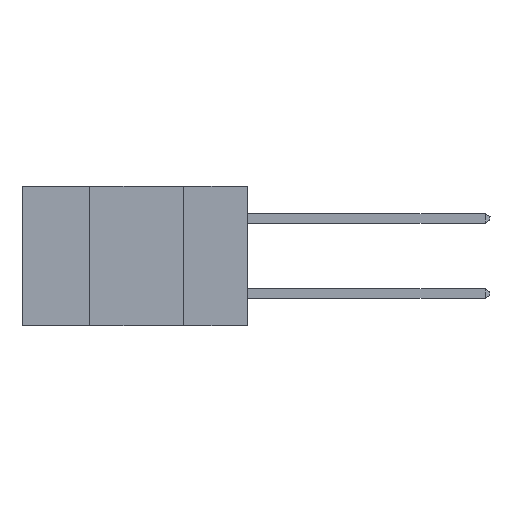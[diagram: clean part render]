
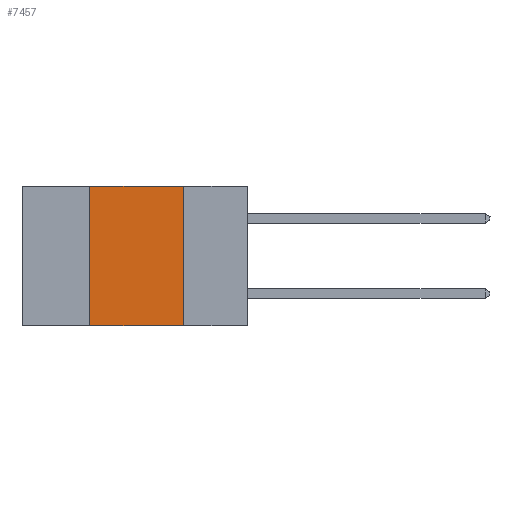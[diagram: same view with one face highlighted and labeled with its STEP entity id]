
A CAD part, left-side view. The second image highlights one B-rep face of the part: STEP entity #7457.
In plain terms, the highlighted planar face has unit normal (-1, 0, 0).
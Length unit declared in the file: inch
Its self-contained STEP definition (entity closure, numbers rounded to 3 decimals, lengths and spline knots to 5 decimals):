
#101 = AXIS2_PLACEMENT_3D ( 'NONE', #11494, #21674, #19981 ) ;
#438 = CARTESIAN_POINT ( 'NONE',  ( 0., 0.17, 0. ) ) ;
#1100 = LINE ( 'NONE', #4126, #12407 ) ;
#1864 = EDGE_CURVE ( 'NONE', #18048, #17075, #9514, .T. ) ;
#1980 = CARTESIAN_POINT ( 'NONE',  ( 0., 0.6, -0.37 ) ) ;
#2754 = CARTESIAN_POINT ( 'NONE',  ( 0., 0.42, 0. ) ) ;
#3656 = LINE ( 'NONE', #1980, #4229 ) ;
#3949 = ORIENTED_EDGE ( 'NONE', *, *, #17112, .F. ) ;
#4126 = CARTESIAN_POINT ( 'NONE',  ( 0., 0.17, -0.37 ) ) ;
#4229 = VECTOR ( 'NONE', #13560, 39.37008 ) ;
#4437 = LINE ( 'NONE', #11219, #6017 ) ;
#4516 = DIRECTION ( 'NONE',  ( 0., 0., 1. ) ) ;
#5463 = ORIENTED_EDGE ( 'NONE', *, *, #1864, .F. ) ;
#6007 = EDGE_LOOP ( 'NONE', ( #10416, #3949, #5463, #12357 ) ) ;
#6017 = VECTOR ( 'NONE', #9327, 39.37008 ) ;
#7457 = ADVANCED_FACE ( 'NONE', ( #10039 ), #13283, .F. ) ;
#9327 = DIRECTION ( 'NONE',  ( 0., -1., 0. ) ) ;
#9514 = LINE ( 'NONE', #19777, #11380 ) ;
#10039 = FACE_OUTER_BOUND ( 'NONE', #6007, .T. ) ;
#10416 = ORIENTED_EDGE ( 'NONE', *, *, #16694, .F. ) ;
#10882 = VERTEX_POINT ( 'NONE', #438 ) ;
#11219 = CARTESIAN_POINT ( 'NONE',  ( 0., 0.6, 0. ) ) ;
#11380 = VECTOR ( 'NONE', #4516, 39.37008 ) ;
#11494 = CARTESIAN_POINT ( 'NONE',  ( 0., 0.6, 0. ) ) ;
#12357 = ORIENTED_EDGE ( 'NONE', *, *, #20001, .T. ) ;
#12407 = VECTOR ( 'NONE', #16019, 39.37008 ) ;
#13151 = VERTEX_POINT ( 'NONE', #21235 ) ;
#13283 = PLANE ( 'NONE',  #101 ) ;
#13560 = DIRECTION ( 'NONE',  ( 0., -1., 0. ) ) ;
#16019 = DIRECTION ( 'NONE',  ( 0., 0., -1. ) ) ;
#16694 = EDGE_CURVE ( 'NONE', #10882, #13151, #1100, .T. ) ;
#17075 = VERTEX_POINT ( 'NONE', #2754 ) ;
#17112 = EDGE_CURVE ( 'NONE', #17075, #10882, #4437, .T. ) ;
#18048 = VERTEX_POINT ( 'NONE', #21335 ) ;
#19777 = CARTESIAN_POINT ( 'NONE',  ( 0., 0.42, -0.37 ) ) ;
#19981 = DIRECTION ( 'NONE',  ( 0., 0., -1. ) ) ;
#20001 = EDGE_CURVE ( 'NONE', #18048, #13151, #3656, .T. ) ;
#21235 = CARTESIAN_POINT ( 'NONE',  ( 0., 0.17, -0.37 ) ) ;
#21335 = CARTESIAN_POINT ( 'NONE',  ( 0., 0.42, -0.37 ) ) ;
#21674 = DIRECTION ( 'NONE',  ( 1., 0., 0. ) ) ;
